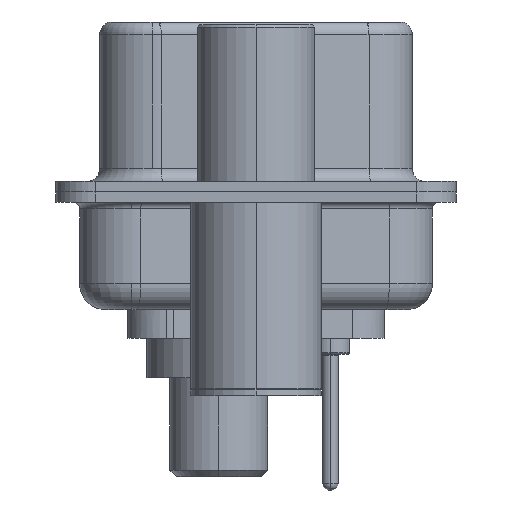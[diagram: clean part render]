
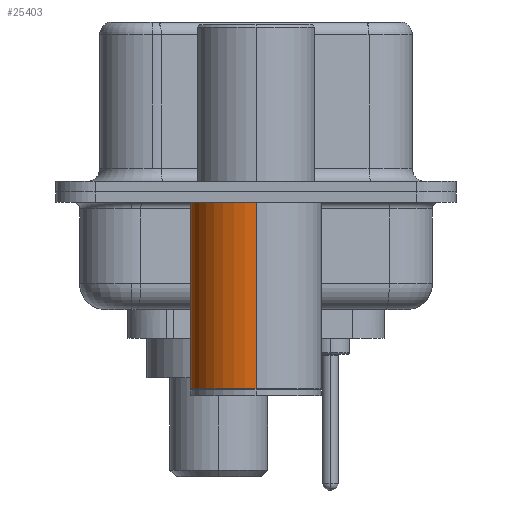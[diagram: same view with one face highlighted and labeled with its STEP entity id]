
A CAD part, left-side view. The second image highlights one B-rep face of the part: STEP entity #25403.
In plain terms, the highlighted cylindrical face has radius 2.5 mm (diameter 5 mm), a partial arc.
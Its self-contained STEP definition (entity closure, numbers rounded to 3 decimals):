
#470 = CARTESIAN_POINT ( 'NONE',  ( 2.5, 0., 0.581 ) ) ;
#1292 = VERTEX_POINT ( 'NONE', #1459 ) ;
#1459 = CARTESIAN_POINT ( 'NONE',  ( 2.5, 0., -7.525 ) ) ;
#4316 = CARTESIAN_POINT ( 'NONE',  ( 0., 0., 0.581 ) ) ;
#5094 = VERTEX_POINT ( 'NONE', #26133 ) ;
#5946 = EDGE_LOOP ( 'NONE', ( #24023, #7169, #6776, #6629 ) ) ;
#5961 = CARTESIAN_POINT ( 'NONE',  ( -2.5, 0., 0.581 ) ) ;
#6586 = AXIS2_PLACEMENT_3D ( 'NONE', #4316, #13028, #21776 ) ;
#6615 = CARTESIAN_POINT ( 'NONE',  ( 0., 0., -0.4 ) ) ;
#6629 = ORIENTED_EDGE ( 'NONE', *, *, #7798, .F. ) ;
#6776 = ORIENTED_EDGE ( 'NONE', *, *, #11995, .F. ) ;
#7169 = ORIENTED_EDGE ( 'NONE', *, *, #10740, .T. ) ;
#7798 = EDGE_CURVE ( 'NONE', #1292, #5094, #11375, .T. ) ;
#8606 = CARTESIAN_POINT ( 'NONE',  ( 0., 0., -7.525 ) ) ;
#8863 = DIRECTION ( 'NONE',  ( 1., 0., 0. ) ) ;
#9068 = EDGE_CURVE ( 'NONE', #1292, #24616, #22576, .T. ) ;
#10066 = CIRCLE ( 'NONE', #25541, 2.5 ) ;
#10740 = EDGE_CURVE ( 'NONE', #24616, #12646, #20757, .T. ) ;
#10796 = DIRECTION ( 'NONE',  ( 1., 0., 0. ) ) ;
#11375 = LINE ( 'NONE', #470, #28086 ) ;
#11995 = EDGE_CURVE ( 'NONE', #5094, #12646, #10066, .T. ) ;
#12186 = DIRECTION ( 'NONE',  ( 0., 0., 1. ) ) ;
#12646 = VERTEX_POINT ( 'NONE', #19706 ) ;
#13028 = DIRECTION ( 'NONE',  ( 0., 0., 1. ) ) ;
#17621 = CARTESIAN_POINT ( 'NONE',  ( -2.5, 0., -7.525 ) ) ;
#19706 = CARTESIAN_POINT ( 'NONE',  ( -2.5, 0., -0.4 ) ) ;
#20757 = LINE ( 'NONE', #5961, #25935 ) ;
#21665 = FACE_OUTER_BOUND ( 'NONE', #5946, .T. ) ;
#21776 = DIRECTION ( 'NONE',  ( 1., 0., 0. ) ) ;
#21880 = DIRECTION ( 'NONE',  ( 0., 0., 1. ) ) ;
#22576 = CIRCLE ( 'NONE', #26222, 2.5 ) ;
#23844 = DIRECTION ( 'NONE',  ( 0., 0., 1. ) ) ;
#24023 = ORIENTED_EDGE ( 'NONE', *, *, #9068, .T. ) ;
#24520 = DIRECTION ( 'NONE',  ( 0., 0., 1. ) ) ;
#24616 = VERTEX_POINT ( 'NONE', #17621 ) ;
#25403 = ADVANCED_FACE ( 'NONE', ( #21665 ), #26829, .T. ) ;
#25541 = AXIS2_PLACEMENT_3D ( 'NONE', #6615, #21880, #8863 ) ;
#25935 = VECTOR ( 'NONE', #12186, 1000. ) ;
#26133 = CARTESIAN_POINT ( 'NONE',  ( 2.5, 0., -0.4 ) ) ;
#26222 = AXIS2_PLACEMENT_3D ( 'NONE', #8606, #23844, #10796 ) ;
#26829 = CYLINDRICAL_SURFACE ( 'NONE', #6586, 2.5 ) ;
#28086 = VECTOR ( 'NONE', #24520, 1000. ) ;
